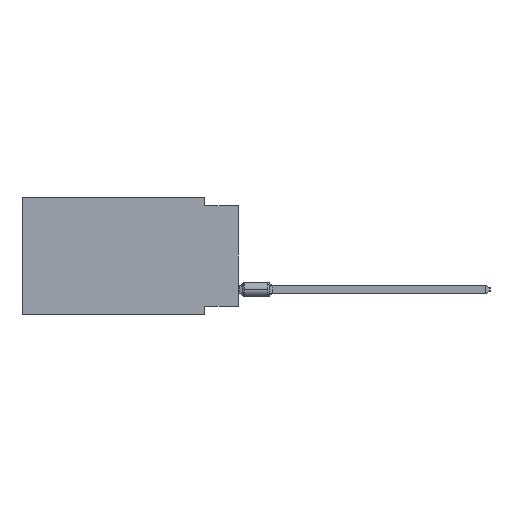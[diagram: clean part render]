
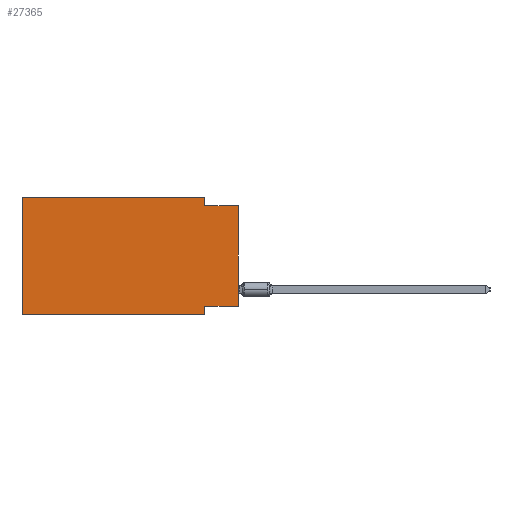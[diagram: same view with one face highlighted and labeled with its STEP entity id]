
A CAD part, left-side view. The second image highlights one B-rep face of the part: STEP entity #27365.
In plain terms, the highlighted planar face has unit normal (-1, 0, 0).
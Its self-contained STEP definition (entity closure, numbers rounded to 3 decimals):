
#36 = ORIENTED_EDGE ( 'NONE', *, *, #26539, .T. ) ;
#386 = ORIENTED_EDGE ( 'NONE', *, *, #22237, .F. ) ;
#408 = DIRECTION ( 'NONE',  ( 0., -1., 0. ) ) ;
#464 = EDGE_CURVE ( 'NONE', #21671, #34526, #12822, .T. ) ;
#820 = ORIENTED_EDGE ( 'NONE', *, *, #10189, .F. ) ;
#924 = VECTOR ( 'NONE', #27472, 1000. ) ;
#2002 = VERTEX_POINT ( 'NONE', #16586 ) ;
#2113 = DIRECTION ( 'NONE',  ( 0., 0., -1. ) ) ;
#3868 = VECTOR ( 'NONE', #4533, 1000. ) ;
#4533 = DIRECTION ( 'NONE',  ( 0., 0., -1. ) ) ;
#4653 = VECTOR ( 'NONE', #10415, 1000. ) ;
#4795 = DIRECTION ( 'NONE',  ( 0., 0., 1. ) ) ;
#4891 = FACE_OUTER_BOUND ( 'NONE', #16953, .T. ) ;
#4913 = CARTESIAN_POINT ( 'NONE',  ( 0., 2.54, 0. ) ) ;
#5202 = ORIENTED_EDGE ( 'NONE', *, *, #31231, .F. ) ;
#5418 = VECTOR ( 'NONE', #15449, 1000. ) ;
#7268 = CARTESIAN_POINT ( 'NONE',  ( 0., 0., -0.635 ) ) ;
#7632 = CARTESIAN_POINT ( 'NONE',  ( 0., 16.383, 0. ) ) ;
#8466 = VECTOR ( 'NONE', #36251, 1000. ) ;
#8898 = DIRECTION ( 'NONE',  ( 0., -1., 0. ) ) ;
#10189 = EDGE_CURVE ( 'NONE', #12744, #15839, #33455, .T. ) ;
#10232 = LINE ( 'NONE', #7268, #4653 ) ;
#10415 = DIRECTION ( 'NONE',  ( 0., -1., 0. ) ) ;
#11234 = AXIS2_PLACEMENT_3D ( 'NONE', #16396, #13061, #2113 ) ;
#12744 = VERTEX_POINT ( 'NONE', #26861 ) ;
#12822 = LINE ( 'NONE', #7632, #924 ) ;
#13061 = DIRECTION ( 'NONE',  ( 1., 0., 0. ) ) ;
#13502 = LINE ( 'NONE', #18890, #34852 ) ;
#14882 = LINE ( 'NONE', #31549, #29556 ) ;
#15101 = EDGE_CURVE ( 'NONE', #21671, #15839, #14882, .T. ) ;
#15449 = DIRECTION ( 'NONE',  ( 0., 1., 0. ) ) ;
#15839 = VERTEX_POINT ( 'NONE', #31093 ) ;
#16396 = CARTESIAN_POINT ( 'NONE',  ( 0., 16.383, 0. ) ) ;
#16586 = CARTESIAN_POINT ( 'NONE',  ( 0., 0., -0.635 ) ) ;
#16953 = EDGE_LOOP ( 'NONE', ( #36, #32276, #386, #27138, #23955, #27399, #820, #5202 ) ) ;
#18890 = CARTESIAN_POINT ( 'NONE',  ( 0., 0., 0. ) ) ;
#19507 = VERTEX_POINT ( 'NONE', #28627 ) ;
#19558 = LINE ( 'NONE', #21805, #3868 ) ;
#20595 = VECTOR ( 'NONE', #8898, 1000. ) ;
#21012 = LINE ( 'NONE', #32290, #5418 ) ;
#21671 = VERTEX_POINT ( 'NONE', #33742 ) ;
#21805 = CARTESIAN_POINT ( 'NONE',  ( 0., 2.54, 0. ) ) ;
#22237 = EDGE_CURVE ( 'NONE', #36492, #35844, #19558, .T. ) ;
#22358 = CARTESIAN_POINT ( 'NONE',  ( 0., 2.54, -8.89 ) ) ;
#22806 = CARTESIAN_POINT ( 'NONE',  ( 0., 16.383, 0. ) ) ;
#23004 = CARTESIAN_POINT ( 'NONE',  ( 0., 16.383, 0. ) ) ;
#23955 = ORIENTED_EDGE ( 'NONE', *, *, #464, .F. ) ;
#24328 = EDGE_CURVE ( 'NONE', #34526, #36492, #27989, .T. ) ;
#26133 = CARTESIAN_POINT ( 'NONE',  ( 0., 2.54, -0.635 ) ) ;
#26539 = EDGE_CURVE ( 'NONE', #19507, #2002, #13502, .T. ) ;
#26861 = CARTESIAN_POINT ( 'NONE',  ( 0., 2.54, -8.255 ) ) ;
#27138 = ORIENTED_EDGE ( 'NONE', *, *, #24328, .F. ) ;
#27365 = ADVANCED_FACE ( 'NONE', ( #4891 ), #36400, .F. ) ;
#27399 = ORIENTED_EDGE ( 'NONE', *, *, #15101, .T. ) ;
#27472 = DIRECTION ( 'NONE',  ( 0., 0., 1. ) ) ;
#27659 = EDGE_CURVE ( 'NONE', #35844, #2002, #10232, .T. ) ;
#27989 = LINE ( 'NONE', #23004, #20595 ) ;
#28627 = CARTESIAN_POINT ( 'NONE',  ( 0., 0., -8.255 ) ) ;
#29556 = VECTOR ( 'NONE', #408, 1000. ) ;
#31093 = CARTESIAN_POINT ( 'NONE',  ( 0., 2.54, -8.89 ) ) ;
#31231 = EDGE_CURVE ( 'NONE', #19507, #12744, #21012, .T. ) ;
#31549 = CARTESIAN_POINT ( 'NONE',  ( 0., 16.383, -8.89 ) ) ;
#32276 = ORIENTED_EDGE ( 'NONE', *, *, #27659, .F. ) ;
#32290 = CARTESIAN_POINT ( 'NONE',  ( 0., 0., -8.255 ) ) ;
#33455 = LINE ( 'NONE', #22358, #8466 ) ;
#33742 = CARTESIAN_POINT ( 'NONE',  ( 0., 16.383, -8.89 ) ) ;
#34526 = VERTEX_POINT ( 'NONE', #22806 ) ;
#34852 = VECTOR ( 'NONE', #4795, 1000. ) ;
#35844 = VERTEX_POINT ( 'NONE', #26133 ) ;
#36251 = DIRECTION ( 'NONE',  ( 0., 0., -1. ) ) ;
#36400 = PLANE ( 'NONE',  #11234 ) ;
#36492 = VERTEX_POINT ( 'NONE', #4913 ) ;
